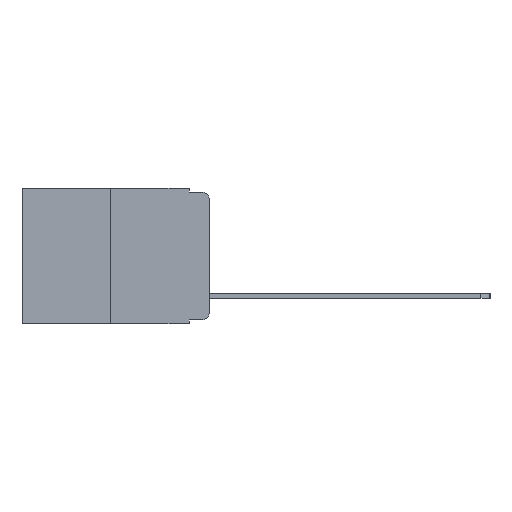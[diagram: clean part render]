
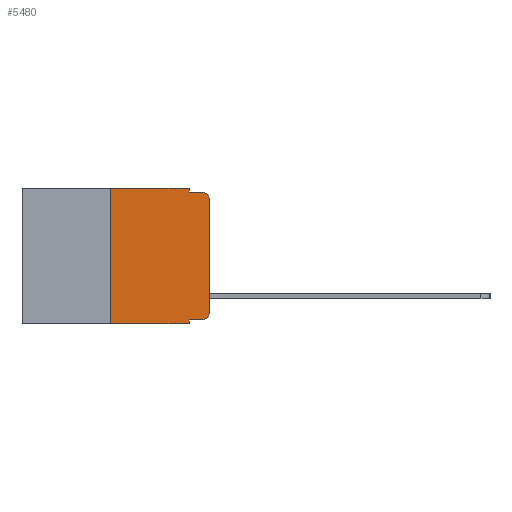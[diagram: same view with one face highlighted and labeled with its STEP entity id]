
A CAD part, left-side view. The second image highlights one B-rep face of the part: STEP entity #5480.
In plain terms, the highlighted planar face has unit normal (-1, 0, 0).
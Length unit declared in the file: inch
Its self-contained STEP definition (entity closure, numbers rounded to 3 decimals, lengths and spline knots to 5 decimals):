
#56 = DIRECTION ( 'NONE',  ( 0., 0., -1. ) ) ;
#779 = CARTESIAN_POINT ( 'NONE',  ( 0., 0.051, -0.333 ) ) ;
#812 = CARTESIAN_POINT ( 'NONE',  ( 0., 0.051, 0. ) ) ;
#1102 = VERTEX_POINT ( 'NONE', #779 ) ;
#1230 = CARTESIAN_POINT ( 'NONE',  ( 0., 0.25, -0.343 ) ) ;
#1246 = LINE ( 'NONE', #3095, #3551 ) ;
#1364 = DIRECTION ( 'NONE',  ( 0., 0., -1. ) ) ;
#1533 = CARTESIAN_POINT ( 'NONE',  ( 0., 0.051, -0.333 ) ) ;
#1568 = DIRECTION ( 'NONE',  ( 0., 0., 1. ) ) ;
#1743 = VERTEX_POINT ( 'NONE', #4127 ) ;
#1758 = VECTOR ( 'NONE', #8477, 39.37008 ) ;
#1802 = VECTOR ( 'NONE', #9235, 39.37008 ) ;
#1804 = CARTESIAN_POINT ( 'NONE',  ( 0., 0.02, -0.01 ) ) ;
#1946 = CARTESIAN_POINT ( 'NONE',  ( 0., 0.051, 0. ) ) ;
#1983 = EDGE_CURVE ( 'NONE', #9862, #4397, #8569, .T. ) ;
#2722 = EDGE_CURVE ( 'NONE', #3648, #9862, #3436, .T. ) ;
#2758 = CARTESIAN_POINT ( 'NONE',  ( 0., 0.473, 0. ) ) ;
#2821 = ORIENTED_EDGE ( 'NONE', *, *, #8027, .F. ) ;
#3095 = CARTESIAN_POINT ( 'NONE',  ( 0., 0.051, -0.01 ) ) ;
#3133 = ORIENTED_EDGE ( 'NONE', *, *, #10908, .T. ) ;
#3343 = VERTEX_POINT ( 'NONE', #7804 ) ;
#3436 = LINE ( 'NONE', #10420, #10304 ) ;
#3551 = VECTOR ( 'NONE', #5106, 39.37008 ) ;
#3648 = VERTEX_POINT ( 'NONE', #5348 ) ;
#3684 = VECTOR ( 'NONE', #10621, 39.37008 ) ;
#4127 = CARTESIAN_POINT ( 'NONE',  ( 0., 0.051, -0.01 ) ) ;
#4303 = LINE ( 'NONE', #1533, #3684 ) ;
#4397 = VERTEX_POINT ( 'NONE', #1804 ) ;
#4558 = AXIS2_PLACEMENT_3D ( 'NONE', #11759, #10164, #4924 ) ;
#4752 = FACE_OUTER_BOUND ( 'NONE', #11570, .T. ) ;
#4875 = AXIS2_PLACEMENT_3D ( 'NONE', #6698, #6754, #8351 ) ;
#4924 = DIRECTION ( 'NONE',  ( 0., 0., -1. ) ) ;
#5090 = DIRECTION ( 'NONE',  ( 0., -1., 0. ) ) ;
#5106 = DIRECTION ( 'NONE',  ( 0., -1., 0. ) ) ;
#5114 = EDGE_CURVE ( 'NONE', #6729, #3648, #6290, .T. ) ;
#5127 = ORIENTED_EDGE ( 'NONE', *, *, #10765, .F. ) ;
#5348 = CARTESIAN_POINT ( 'NONE',  ( 0., 0., -0.313 ) ) ;
#5431 = ORIENTED_EDGE ( 'NONE', *, *, #8578, .T. ) ;
#5480 = ADVANCED_FACE ( 'NONE', ( #4752 ), #9373, .F. ) ;
#5804 = EDGE_CURVE ( 'NONE', #3343, #7273, #11130, .T. ) ;
#5962 = DIRECTION ( 'NONE',  ( -1., 0., 0. ) ) ;
#6223 = VERTEX_POINT ( 'NONE', #7905 ) ;
#6225 = VECTOR ( 'NONE', #5090, 39.37008 ) ;
#6290 = CIRCLE ( 'NONE', #11269, 0.02 ) ;
#6579 = CARTESIAN_POINT ( 'NONE',  ( 0., 0.25, 0. ) ) ;
#6646 = LINE ( 'NONE', #812, #1758 ) ;
#6698 = CARTESIAN_POINT ( 'NONE',  ( 0., 0.02, -0.03 ) ) ;
#6729 = VERTEX_POINT ( 'NONE', #8204 ) ;
#6754 = DIRECTION ( 'NONE',  ( -1., 0., 0. ) ) ;
#6812 = VECTOR ( 'NONE', #7523, 39.37008 ) ;
#7219 = CARTESIAN_POINT ( 'NONE',  ( 0., 0.051, 0. ) ) ;
#7273 = VERTEX_POINT ( 'NONE', #1946 ) ;
#7363 = ORIENTED_EDGE ( 'NONE', *, *, #1983, .T. ) ;
#7523 = DIRECTION ( 'NONE',  ( 0., 0., 1. ) ) ;
#7607 = CARTESIAN_POINT ( 'NONE',  ( 0., 0., -0.03 ) ) ;
#7647 = ORIENTED_EDGE ( 'NONE', *, *, #5804, .F. ) ;
#7676 = VERTEX_POINT ( 'NONE', #1230 ) ;
#7752 = LINE ( 'NONE', #7219, #9671 ) ;
#7804 = CARTESIAN_POINT ( 'NONE',  ( 0., 0.25, 0. ) ) ;
#7905 = CARTESIAN_POINT ( 'NONE',  ( 0., 0.051, -0.343 ) ) ;
#8027 = EDGE_CURVE ( 'NONE', #7676, #3343, #9105, .T. ) ;
#8186 = ORIENTED_EDGE ( 'NONE', *, *, #5114, .T. ) ;
#8204 = CARTESIAN_POINT ( 'NONE',  ( 0., 0.02, -0.333 ) ) ;
#8291 = EDGE_CURVE ( 'NONE', #1102, #6223, #6646, .T. ) ;
#8351 = DIRECTION ( 'NONE',  ( 0., 0., -1. ) ) ;
#8477 = DIRECTION ( 'NONE',  ( 0., 0., -1. ) ) ;
#8569 = CIRCLE ( 'NONE', #4875, 0.02 ) ;
#8578 = EDGE_CURVE ( 'NONE', #7676, #6223, #8588, .T. ) ;
#8588 = LINE ( 'NONE', #10306, #6225 ) ;
#9105 = LINE ( 'NONE', #6579, #6812 ) ;
#9235 = DIRECTION ( 'NONE',  ( 0., -1., 0. ) ) ;
#9308 = ORIENTED_EDGE ( 'NONE', *, *, #2722, .T. ) ;
#9373 = PLANE ( 'NONE',  #4558 ) ;
#9570 = ORIENTED_EDGE ( 'NONE', *, *, #10159, .F. ) ;
#9671 = VECTOR ( 'NONE', #1364, 39.37008 ) ;
#9862 = VERTEX_POINT ( 'NONE', #7607 ) ;
#10048 = ORIENTED_EDGE ( 'NONE', *, *, #8291, .F. ) ;
#10159 = EDGE_CURVE ( 'NONE', #1743, #4397, #1246, .T. ) ;
#10164 = DIRECTION ( 'NONE',  ( 1., 0., 0. ) ) ;
#10304 = VECTOR ( 'NONE', #1568, 39.37008 ) ;
#10306 = CARTESIAN_POINT ( 'NONE',  ( 0., 0.473, -0.343 ) ) ;
#10420 = CARTESIAN_POINT ( 'NONE',  ( 0., 0., 0. ) ) ;
#10621 = DIRECTION ( 'NONE',  ( 0., -1., 0. ) ) ;
#10765 = EDGE_CURVE ( 'NONE', #7273, #1743, #7752, .T. ) ;
#10908 = EDGE_CURVE ( 'NONE', #1102, #6729, #4303, .T. ) ;
#11041 = CARTESIAN_POINT ( 'NONE',  ( 0., 0.02, -0.313 ) ) ;
#11130 = LINE ( 'NONE', #2758, #1802 ) ;
#11269 = AXIS2_PLACEMENT_3D ( 'NONE', #11041, #5962, #56 ) ;
#11570 = EDGE_LOOP ( 'NONE', ( #9308, #7363, #9570, #5127, #7647, #2821, #5431, #10048, #3133, #8186 ) ) ;
#11759 = CARTESIAN_POINT ( 'NONE',  ( 0., 0.473, 0. ) ) ;
